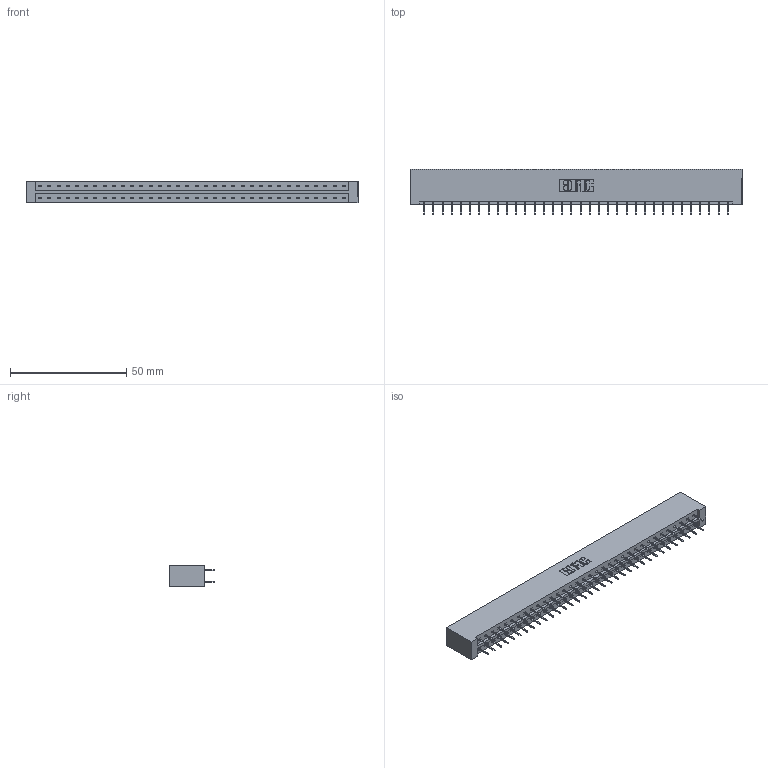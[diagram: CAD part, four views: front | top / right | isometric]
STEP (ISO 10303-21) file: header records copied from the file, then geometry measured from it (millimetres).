
FILE_DESCRIPTION (( 'STEP AP203' ), '1' );
FILE_NAME ('833-068-524-201.STEP', '2020-06-05T10:25:13', ( '' ), ( '' ), 'SwSTEP 2.0', 'SolidWorks 2020', '' );
FILE_SCHEMA (( 'CONFIG_CONTROL_DESIGN' ));
Length unit declared in the file: inch
Products named in the file (3): 345-292-001_345-293-124; 833 Part_Lugless; 833-068-524-201
Assembly tree (69 placements, depth 2):
  833-068-524-201
    833 Part_Lugless
    345-292-001_345-293-124  x68
Bounding box: 142.98 x 19.69 x 9.4 mm (x, y, z)
Volume: 15051.6 mm3; surface area: 17424.3 mm2
Topology: 69 solids, 69 shells, 3914 faces, 11099 edges, 7126 vertices
Faces by surface type: plane 2922, cylinder 992
Entity records: 22705 total; most frequent: CARTESIAN_POINT 3770, ORIENTED_EDGE 3706, DIRECTION 3229, EDGE_CURVE 1853, LINE 1737, VECTOR 1737, VERTEX_POINT 1230, AXIS2_PLACEMENT_3D 746
